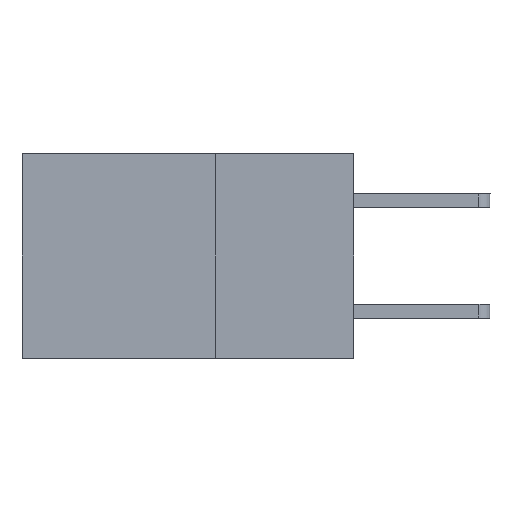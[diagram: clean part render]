
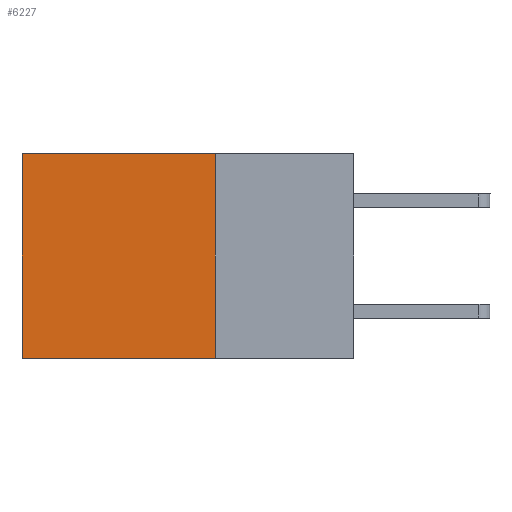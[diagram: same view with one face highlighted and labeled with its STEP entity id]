
A CAD part, left-side view. The second image highlights one B-rep face of the part: STEP entity #6227.
In plain terms, the highlighted planar face has unit normal (-1, 0, 0).
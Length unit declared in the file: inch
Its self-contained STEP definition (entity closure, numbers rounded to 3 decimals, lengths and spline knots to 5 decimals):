
#250 = EDGE_CURVE ( 'NONE', #2019, #9545, #1169, .T. ) ;
#469 = CARTESIAN_POINT ( 'NONE',  ( 0.2875, 0.25, 0. ) ) ;
#666 = EDGE_CURVE ( 'NONE', #9545, #2735, #5500, .T. ) ;
#684 = CARTESIAN_POINT ( 'NONE',  ( 0.2875, 0.25, -0.37 ) ) ;
#1169 = LINE ( 'NONE', #469, #5364 ) ;
#1624 = CARTESIAN_POINT ( 'NONE',  ( 0.2875, 0.6, 0. ) ) ;
#1660 = CARTESIAN_POINT ( 'NONE',  ( 0.2875, 0.25, 0. ) ) ;
#2019 = VERTEX_POINT ( 'NONE', #1660 ) ;
#2030 = VERTEX_POINT ( 'NONE', #1624 ) ;
#2270 = EDGE_CURVE ( 'NONE', #2030, #2735, #8632, .T. ) ;
#2735 = VERTEX_POINT ( 'NONE', #4778 ) ;
#3015 = CARTESIAN_POINT ( 'NONE',  ( 0.2875, 0.25, 0. ) ) ;
#3053 = ORIENTED_EDGE ( 'NONE', *, *, #250, .F. ) ;
#3121 = ORIENTED_EDGE ( 'NONE', *, *, #2270, .T. ) ;
#3467 = VECTOR ( 'NONE', #4651, 39.37008 ) ;
#3546 = ORIENTED_EDGE ( 'NONE', *, *, #666, .F. ) ;
#3778 = DIRECTION ( 'NONE',  ( 1., 0., 0. ) ) ;
#4264 = ORIENTED_EDGE ( 'NONE', *, *, #9008, .T. ) ;
#4651 = DIRECTION ( 'NONE',  ( 0., 1., 0. ) ) ;
#4756 = CARTESIAN_POINT ( 'NONE',  ( 0.2875, 0.25, -0.37 ) ) ;
#4778 = CARTESIAN_POINT ( 'NONE',  ( 0.2875, 0.6, -0.37 ) ) ;
#4825 = DIRECTION ( 'NONE',  ( 0., 1., 0. ) ) ;
#4881 = VECTOR ( 'NONE', #4921, 39.37008 ) ;
#4921 = DIRECTION ( 'NONE',  ( 0., 0., -1. ) ) ;
#5364 = VECTOR ( 'NONE', #9367, 39.37008 ) ;
#5409 = EDGE_LOOP ( 'NONE', ( #3121, #3546, #3053, #4264 ) ) ;
#5500 = LINE ( 'NONE', #4756, #3467 ) ;
#6227 = ADVANCED_FACE ( 'NONE', ( #8338 ), #7550, .F. ) ;
#6886 = LINE ( 'NONE', #8568, #8619 ) ;
#7550 = PLANE ( 'NONE',  #9342 ) ;
#8338 = FACE_OUTER_BOUND ( 'NONE', #5409, .T. ) ;
#8568 = CARTESIAN_POINT ( 'NONE',  ( 0.2875, 0.25, 0. ) ) ;
#8619 = VECTOR ( 'NONE', #4825, 39.37008 ) ;
#8632 = LINE ( 'NONE', #9391, #4881 ) ;
#9008 = EDGE_CURVE ( 'NONE', #2019, #2030, #6886, .T. ) ;
#9037 = DIRECTION ( 'NONE',  ( 0., 0., -1. ) ) ;
#9342 = AXIS2_PLACEMENT_3D ( 'NONE', #3015, #3778, #9037 ) ;
#9367 = DIRECTION ( 'NONE',  ( 0., 0., -1. ) ) ;
#9391 = CARTESIAN_POINT ( 'NONE',  ( 0.2875, 0.6, 0. ) ) ;
#9545 = VERTEX_POINT ( 'NONE', #684 ) ;
